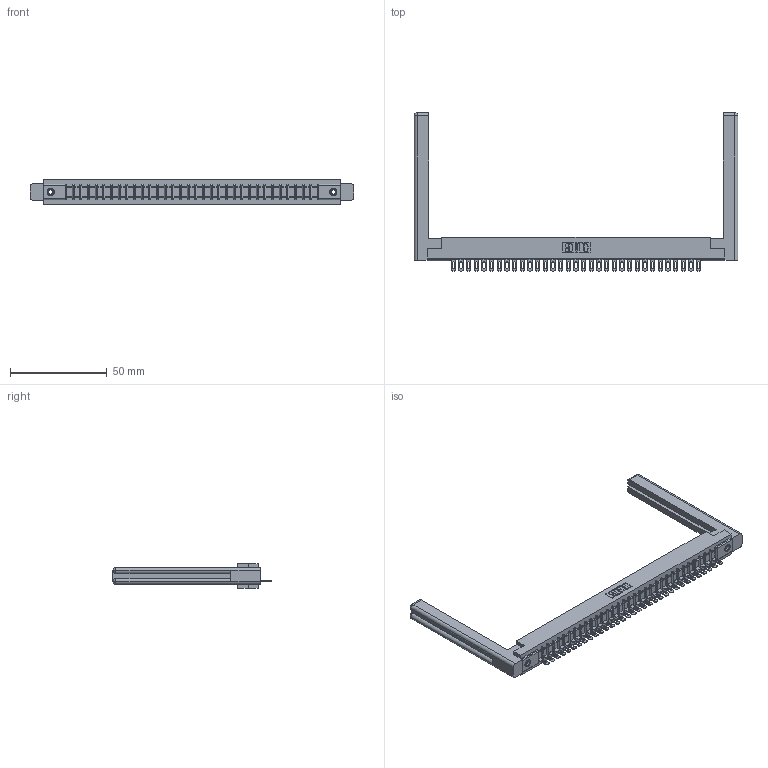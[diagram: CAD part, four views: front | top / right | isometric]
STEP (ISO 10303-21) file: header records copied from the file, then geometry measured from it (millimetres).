
FILE_DESCRIPTION (( 'STEP AP203' ), '1' );
FILE_NAME ('307-033-501-158.STEP', '2019-09-05T05:47:38', ( '' ), ( '' ), 'SwSTEP 2.0', 'SolidWorks 2016', '' );
FILE_SCHEMA (( 'CONFIG_CONTROL_DESIGN' ));
Length unit declared in the file: inch
Products named in the file (5): 307-290-002_501; 307-220-058; 307-033-501-158; 307 Part_.156 Dia Mounting Holes; 345-250-001_345-250-001-102
Assembly tree (38 placements, depth 2):
  307-033-501-158
    307 Part_.156 Dia Mounting Holes
    307-290-002_501  x33
    307-220-058  x2
    345-250-001_345-250-001-102  x2
Bounding box: 167.39 x 81.74 x 12.7 mm (x, y, z)
Volume: 24994.3 mm3; surface area: 27331.8 mm2
Topology: 38 solids, 38 shells, 2802 faces, 8531 edges, 5582 vertices
Faces by surface type: plane 1606, cylinder 1104, sphere 68, torus 12, cone 12
Entity records: 32827 total; most frequent: CARTESIAN_POINT 5543, ORIENTED_EDGE 5472, DIRECTION 5354, EDGE_CURVE 2736, VECTOR 2084, LINE 2084, VERTEX_POINT 1770, AXIS2_PLACEMENT_3D 1635
